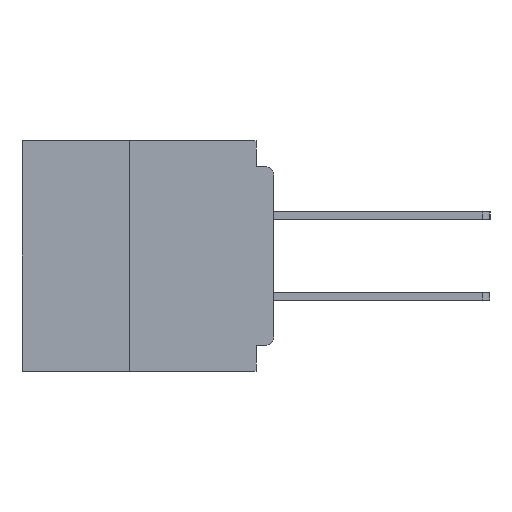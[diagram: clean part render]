
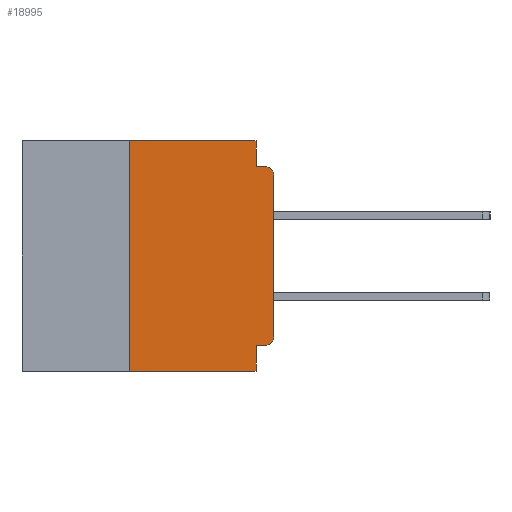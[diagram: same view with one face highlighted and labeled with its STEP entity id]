
A CAD part, left-side view. The second image highlights one B-rep face of the part: STEP entity #18995.
In plain terms, the highlighted planar face has unit normal (-1, 0, 0).
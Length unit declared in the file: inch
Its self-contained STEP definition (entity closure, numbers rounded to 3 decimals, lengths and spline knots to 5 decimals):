
#982 = VECTOR ( 'NONE', #41735, 39.37008 ) ;
#1494 = ORIENTED_EDGE ( 'NONE', *, *, #12183, .F. ) ;
#1687 = DIRECTION ( 'NONE',  ( 0., 0., -1. ) ) ;
#1900 = LINE ( 'NONE', #40289, #39990 ) ;
#1958 = DIRECTION ( 'NONE',  ( 0., -1., 0. ) ) ;
#2134 = FACE_OUTER_BOUND ( 'NONE', #38897, .T. ) ;
#2661 = EDGE_CURVE ( 'NONE', #10760, #16033, #29396, .T. ) ;
#2896 = CARTESIAN_POINT ( 'NONE',  ( 0., 0.437, 0. ) ) ;
#3345 = DIRECTION ( 'NONE',  ( 0., 0., -1. ) ) ;
#5228 = CARTESIAN_POINT ( 'NONE',  ( 0., 0.015, -0.355 ) ) ;
#6014 = EDGE_CURVE ( 'NONE', #43744, #31881, #21030, .T. ) ;
#6131 = ORIENTED_EDGE ( 'NONE', *, *, #40027, .F. ) ;
#6642 = ORIENTED_EDGE ( 'NONE', *, *, #34010, .T. ) ;
#7196 = CARTESIAN_POINT ( 'NONE',  ( 0., 0.031, 0. ) ) ;
#7198 = DIRECTION ( 'NONE',  ( 0., 0., 1. ) ) ;
#8792 = DIRECTION ( 'NONE',  ( 0., 0., -1. ) ) ;
#8795 = AXIS2_PLACEMENT_3D ( 'NONE', #47451, #25475, #3345 ) ;
#9848 = DIRECTION ( 'NONE',  ( -1., 0., 0. ) ) ;
#10198 = ORIENTED_EDGE ( 'NONE', *, *, #28736, .T. ) ;
#10760 = VERTEX_POINT ( 'NONE', #5228 ) ;
#11341 = VERTEX_POINT ( 'NONE', #38542 ) ;
#12088 = CARTESIAN_POINT ( 'NONE',  ( 0., 0., -0.06 ) ) ;
#12089 = VERTEX_POINT ( 'NONE', #12088 ) ;
#12183 = EDGE_CURVE ( 'NONE', #35927, #33724, #30081, .T. ) ;
#12493 = CARTESIAN_POINT ( 'NONE',  ( 0., 0., -0.34 ) ) ;
#12733 = VECTOR ( 'NONE', #27126, 39.37008 ) ;
#12829 = AXIS2_PLACEMENT_3D ( 'NONE', #2896, #39978, #17956 ) ;
#13105 = ORIENTED_EDGE ( 'NONE', *, *, #2661, .T. ) ;
#13662 = LINE ( 'NONE', #20356, #40662 ) ;
#14810 = ORIENTED_EDGE ( 'NONE', *, *, #6014, .F. ) ;
#16033 = VERTEX_POINT ( 'NONE', #12493 ) ;
#16072 = CARTESIAN_POINT ( 'NONE',  ( 0., 0.031, 0. ) ) ;
#17956 = DIRECTION ( 'NONE',  ( 0., 0., -1. ) ) ;
#18995 = ADVANCED_FACE ( 'NONE', ( #2134 ), #36290, .F. ) ;
#19369 = CARTESIAN_POINT ( 'NONE',  ( 0., 0.031, -0.045 ) ) ;
#19626 = VERTEX_POINT ( 'NONE', #47111 ) ;
#19711 = CARTESIAN_POINT ( 'NONE',  ( 0., 0., 0. ) ) ;
#20356 = CARTESIAN_POINT ( 'NONE',  ( 0., 0., -0.355 ) ) ;
#21030 = LINE ( 'NONE', #16072, #29640 ) ;
#23655 = VECTOR ( 'NONE', #7198, 39.37008 ) ;
#24041 = DIRECTION ( 'NONE',  ( 0., 1., 0. ) ) ;
#24639 = ORIENTED_EDGE ( 'NONE', *, *, #47634, .F. ) ;
#25475 = DIRECTION ( 'NONE',  ( -1., 0., 0. ) ) ;
#25552 = VERTEX_POINT ( 'NONE', #45273 ) ;
#26984 = EDGE_CURVE ( 'NONE', #16033, #12089, #42073, .T. ) ;
#27126 = DIRECTION ( 'NONE',  ( 0., 0., 1. ) ) ;
#28047 = ORIENTED_EDGE ( 'NONE', *, *, #37897, .F. ) ;
#28736 = EDGE_CURVE ( 'NONE', #25552, #33724, #30459, .T. ) ;
#29396 = CIRCLE ( 'NONE', #8795, 0.015 ) ;
#29640 = VECTOR ( 'NONE', #8792, 39.37008 ) ;
#29840 = VECTOR ( 'NONE', #1958, 39.37008 ) ;
#30081 = LINE ( 'NONE', #45816, #47325 ) ;
#30459 = LINE ( 'NONE', #38050, #982 ) ;
#30607 = CARTESIAN_POINT ( 'NONE',  ( 0., 0.031, -0.355 ) ) ;
#31490 = ORIENTED_EDGE ( 'NONE', *, *, #35701, .F. ) ;
#31881 = VERTEX_POINT ( 'NONE', #19369 ) ;
#31923 = CARTESIAN_POINT ( 'NONE',  ( 0., 0.015, -0.06 ) ) ;
#33724 = VERTEX_POINT ( 'NONE', #41392 ) ;
#34010 = EDGE_CURVE ( 'NONE', #12089, #19626, #45797, .T. ) ;
#34606 = LINE ( 'NONE', #36520, #23655 ) ;
#35619 = DIRECTION ( 'NONE',  ( 0., 0., -1. ) ) ;
#35701 = EDGE_CURVE ( 'NONE', #31881, #19626, #1900, .T. ) ;
#35927 = VERTEX_POINT ( 'NONE', #30607 ) ;
#36290 = PLANE ( 'NONE',  #12829 ) ;
#36520 = CARTESIAN_POINT ( 'NONE',  ( 0., 0.25, -0.4 ) ) ;
#37897 = EDGE_CURVE ( 'NONE', #25552, #11341, #34606, .T. ) ;
#38050 = CARTESIAN_POINT ( 'NONE',  ( 0., 0.437, -0.4 ) ) ;
#38542 = CARTESIAN_POINT ( 'NONE',  ( 0., 0.25, 0. ) ) ;
#38897 = EDGE_LOOP ( 'NONE', ( #43496, #6642, #31490, #14810, #6131, #28047, #10198, #1494, #24639, #13105 ) ) ;
#39645 = LINE ( 'NONE', #46088, #29840 ) ;
#39978 = DIRECTION ( 'NONE',  ( 1., 0., 0. ) ) ;
#39990 = VECTOR ( 'NONE', #47629, 39.37008 ) ;
#40027 = EDGE_CURVE ( 'NONE', #11341, #43744, #39645, .T. ) ;
#40289 = CARTESIAN_POINT ( 'NONE',  ( 0., 0., -0.045 ) ) ;
#40662 = VECTOR ( 'NONE', #24041, 39.37008 ) ;
#41392 = CARTESIAN_POINT ( 'NONE',  ( 0., 0.031, -0.4 ) ) ;
#41735 = DIRECTION ( 'NONE',  ( 0., -1., 0. ) ) ;
#41892 = AXIS2_PLACEMENT_3D ( 'NONE', #31923, #9848, #35619 ) ;
#42073 = LINE ( 'NONE', #19711, #12733 ) ;
#43496 = ORIENTED_EDGE ( 'NONE', *, *, #26984, .T. ) ;
#43744 = VERTEX_POINT ( 'NONE', #7196 ) ;
#45273 = CARTESIAN_POINT ( 'NONE',  ( 0., 0.25, -0.4 ) ) ;
#45797 = CIRCLE ( 'NONE', #41892, 0.015 ) ;
#45816 = CARTESIAN_POINT ( 'NONE',  ( 0., 0.031, -0.4 ) ) ;
#46088 = CARTESIAN_POINT ( 'NONE',  ( 0., 0.437, 0. ) ) ;
#47111 = CARTESIAN_POINT ( 'NONE',  ( 0., 0.015, -0.045 ) ) ;
#47325 = VECTOR ( 'NONE', #1687, 39.37008 ) ;
#47451 = CARTESIAN_POINT ( 'NONE',  ( 0., 0.015, -0.34 ) ) ;
#47629 = DIRECTION ( 'NONE',  ( 0., -1., 0. ) ) ;
#47634 = EDGE_CURVE ( 'NONE', #10760, #35927, #13662, .T. ) ;
